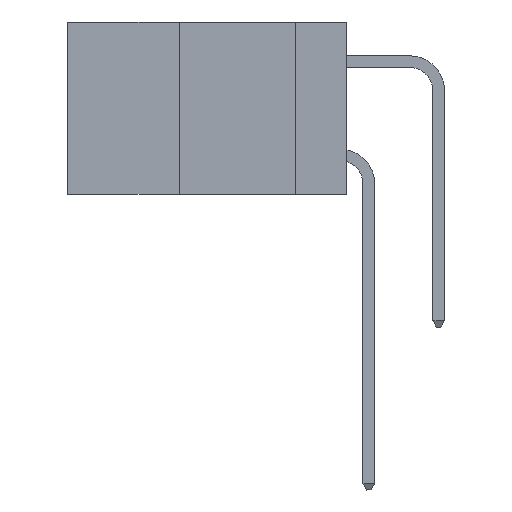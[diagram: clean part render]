
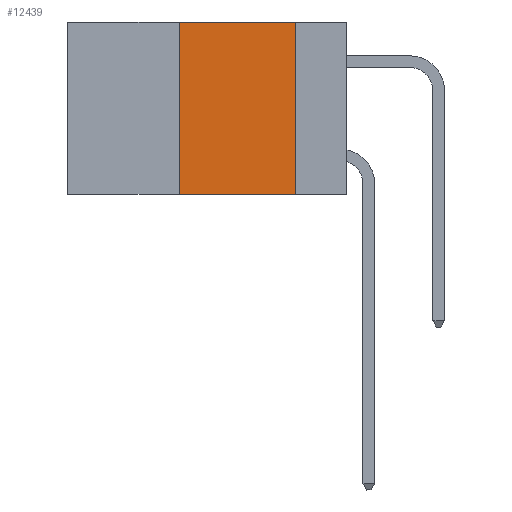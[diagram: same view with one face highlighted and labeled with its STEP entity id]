
A CAD part, left-side view. The second image highlights one B-rep face of the part: STEP entity #12439.
In plain terms, the highlighted planar face has unit normal (-1, 0, 0).
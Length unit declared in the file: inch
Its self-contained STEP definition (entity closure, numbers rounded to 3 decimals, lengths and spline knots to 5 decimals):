
#222 = DIRECTION ( 'NONE',  ( 0., -1., 0. ) ) ;
#547 = DIRECTION ( 'NONE',  ( 0., 0., -1. ) ) ;
#2154 = EDGE_CURVE ( 'NONE', #33038, #10133, #27182, .T. ) ;
#3504 = CARTESIAN_POINT ( 'NONE',  ( 0., 0.11, 0. ) ) ;
#4053 = CARTESIAN_POINT ( 'NONE',  ( 0., 0.11, -0.37 ) ) ;
#5449 = VECTOR ( 'NONE', #25228, 39.37008 ) ;
#5499 = CARTESIAN_POINT ( 'NONE',  ( 0., 0.6, 0. ) ) ;
#6247 = EDGE_LOOP ( 'NONE', ( #8724, #21057, #29170, #8915 ) ) ;
#8362 = DIRECTION ( 'NONE',  ( 0., 0., 1. ) ) ;
#8565 = CARTESIAN_POINT ( 'NONE',  ( 0., 0.11, 0. ) ) ;
#8724 = ORIENTED_EDGE ( 'NONE', *, *, #11533, .F. ) ;
#8915 = ORIENTED_EDGE ( 'NONE', *, *, #2154, .T. ) ;
#10133 = VERTEX_POINT ( 'NONE', #4053 ) ;
#10295 = EDGE_CURVE ( 'NONE', #28288, #22824, #28110, .T. ) ;
#10829 = DIRECTION ( 'NONE',  ( 1., 0., 0. ) ) ;
#11533 = EDGE_CURVE ( 'NONE', #22824, #10133, #25912, .T. ) ;
#12439 = ADVANCED_FACE ( 'NONE', ( #13054 ), #21467, .F. ) ;
#13054 = FACE_OUTER_BOUND ( 'NONE', #6247, .T. ) ;
#17012 = CARTESIAN_POINT ( 'NONE',  ( 0., 0.36, 0. ) ) ;
#17380 = DIRECTION ( 'NONE',  ( 0., 0., -1. ) ) ;
#20814 = CARTESIAN_POINT ( 'NONE',  ( 0., 0.36, -0.37 ) ) ;
#21057 = ORIENTED_EDGE ( 'NONE', *, *, #10295, .F. ) ;
#21238 = VECTOR ( 'NONE', #17380, 39.37008 ) ;
#21467 = PLANE ( 'NONE',  #33871 ) ;
#21499 = CARTESIAN_POINT ( 'NONE',  ( 0., 0.36, 0. ) ) ;
#21723 = VECTOR ( 'NONE', #222, 39.37008 ) ;
#22824 = VERTEX_POINT ( 'NONE', #8565 ) ;
#25228 = DIRECTION ( 'NONE',  ( 0., -1., 0. ) ) ;
#25912 = LINE ( 'NONE', #3504, #21238 ) ;
#27182 = LINE ( 'NONE', #30219, #5449 ) ;
#27238 = CARTESIAN_POINT ( 'NONE',  ( 0., 0.6, 0. ) ) ;
#28110 = LINE ( 'NONE', #27238, #21723 ) ;
#28288 = VERTEX_POINT ( 'NONE', #21499 ) ;
#28540 = VECTOR ( 'NONE', #8362, 39.37008 ) ;
#29170 = ORIENTED_EDGE ( 'NONE', *, *, #29261, .F. ) ;
#29261 = EDGE_CURVE ( 'NONE', #33038, #28288, #29432, .T. ) ;
#29432 = LINE ( 'NONE', #17012, #28540 ) ;
#30219 = CARTESIAN_POINT ( 'NONE',  ( 0., 0.6, -0.37 ) ) ;
#33038 = VERTEX_POINT ( 'NONE', #20814 ) ;
#33871 = AXIS2_PLACEMENT_3D ( 'NONE', #5499, #10829, #547 ) ;
